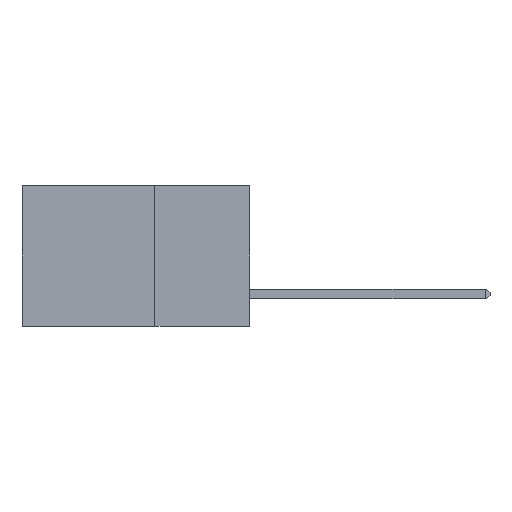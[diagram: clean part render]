
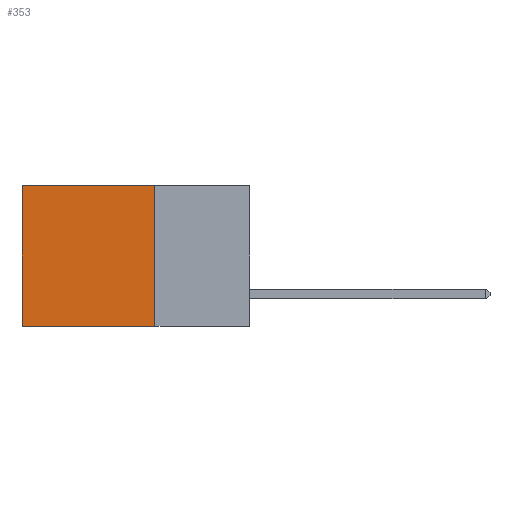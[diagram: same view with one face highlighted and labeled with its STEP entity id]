
A CAD part, left-side view. The second image highlights one B-rep face of the part: STEP entity #353.
In plain terms, the highlighted planar face has unit normal (-1, 0, 0).
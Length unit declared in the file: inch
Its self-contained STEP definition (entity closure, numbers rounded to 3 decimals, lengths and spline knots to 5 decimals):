
#353 = ADVANCED_FACE ( 'NONE', ( #3335 ), #8336, .F. ) ;
#435 = DIRECTION ( 'NONE',  ( 0., 1., 0. ) ) ;
#456 = CARTESIAN_POINT ( 'NONE',  ( 0.2875, 0.6, 0. ) ) ;
#538 = CARTESIAN_POINT ( 'NONE',  ( 0.2875, 0.25, 0. ) ) ;
#848 = VECTOR ( 'NONE', #1193, 39.37008 ) ;
#1193 = DIRECTION ( 'NONE',  ( 0., 0., -1. ) ) ;
#1196 = VERTEX_POINT ( 'NONE', #7652 ) ;
#1386 = CARTESIAN_POINT ( 'NONE',  ( 0.2875, 0.6, 0. ) ) ;
#1401 = EDGE_CURVE ( 'NONE', #5583, #1196, #8174, .T. ) ;
#1549 = DIRECTION ( 'NONE',  ( 0., 0., -1. ) ) ;
#2050 = ORIENTED_EDGE ( 'NONE', *, *, #5106, .T. ) ;
#2703 = ORIENTED_EDGE ( 'NONE', *, *, #9174, .F. ) ;
#2707 = AXIS2_PLACEMENT_3D ( 'NONE', #4907, #9561, #11041 ) ;
#3335 = FACE_OUTER_BOUND ( 'NONE', #6981, .T. ) ;
#3566 = LINE ( 'NONE', #1386, #848 ) ;
#3933 = VECTOR ( 'NONE', #1549, 39.37008 ) ;
#4287 = CARTESIAN_POINT ( 'NONE',  ( 0.2875, 0.25, 0. ) ) ;
#4907 = CARTESIAN_POINT ( 'NONE',  ( 0.2875, 0.25, 0. ) ) ;
#5052 = ORIENTED_EDGE ( 'NONE', *, *, #1401, .F. ) ;
#5106 = EDGE_CURVE ( 'NONE', #7137, #1196, #3566, .T. ) ;
#5216 = VERTEX_POINT ( 'NONE', #4287 ) ;
#5583 = VERTEX_POINT ( 'NONE', #10804 ) ;
#6577 = DIRECTION ( 'NONE',  ( 0., 1., 0. ) ) ;
#6845 = CARTESIAN_POINT ( 'NONE',  ( 0.2875, 0.25, -0.37 ) ) ;
#6981 = EDGE_LOOP ( 'NONE', ( #2050, #5052, #2703, #7934 ) ) ;
#7137 = VERTEX_POINT ( 'NONE', #456 ) ;
#7567 = LINE ( 'NONE', #11770, #11920 ) ;
#7652 = CARTESIAN_POINT ( 'NONE',  ( 0.2875, 0.6, -0.37 ) ) ;
#7934 = ORIENTED_EDGE ( 'NONE', *, *, #11626, .T. ) ;
#8174 = LINE ( 'NONE', #6845, #10755 ) ;
#8336 = PLANE ( 'NONE',  #2707 ) ;
#9174 = EDGE_CURVE ( 'NONE', #5216, #5583, #11554, .T. ) ;
#9561 = DIRECTION ( 'NONE',  ( 1., 0., 0. ) ) ;
#10755 = VECTOR ( 'NONE', #6577, 39.37008 ) ;
#10804 = CARTESIAN_POINT ( 'NONE',  ( 0.2875, 0.25, -0.37 ) ) ;
#11041 = DIRECTION ( 'NONE',  ( 0., 0., -1. ) ) ;
#11554 = LINE ( 'NONE', #538, #3933 ) ;
#11626 = EDGE_CURVE ( 'NONE', #5216, #7137, #7567, .T. ) ;
#11770 = CARTESIAN_POINT ( 'NONE',  ( 0.2875, 0.25, 0. ) ) ;
#11920 = VECTOR ( 'NONE', #435, 39.37008 ) ;
